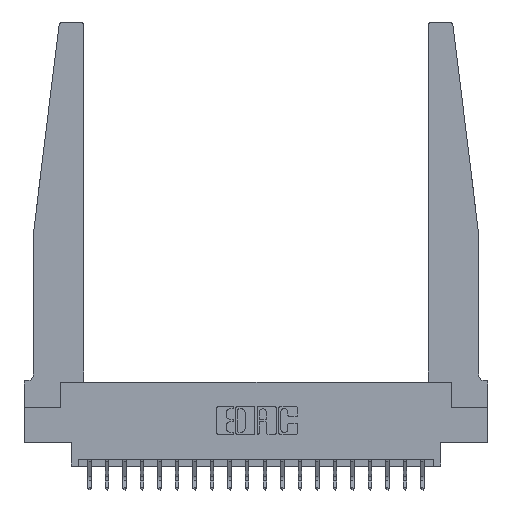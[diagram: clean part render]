
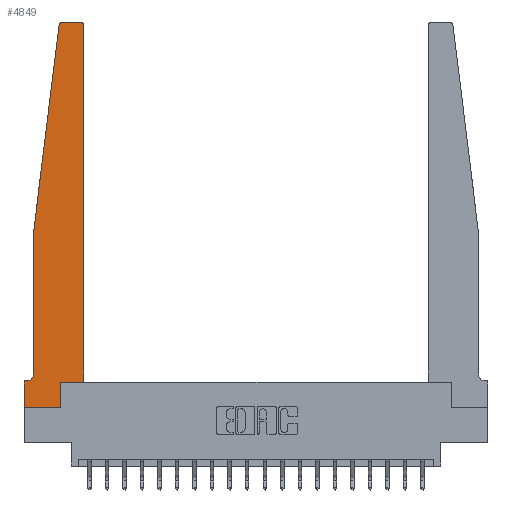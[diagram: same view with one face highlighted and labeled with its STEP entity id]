
A CAD part, top view. The second image highlights one B-rep face of the part: STEP entity #4849.
In plain terms, the highlighted planar face has unit normal (0, 0, 1).
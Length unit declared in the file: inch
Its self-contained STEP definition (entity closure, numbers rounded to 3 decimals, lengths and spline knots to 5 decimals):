
#12 = VERTEX_POINT ( 'NONE', #3323 ) ;
#208 = DIRECTION ( 'NONE',  ( -1., 0., 0. ) ) ;
#365 = VECTOR ( 'NONE', #12422, 39.37008 ) ;
#427 = LINE ( 'NONE', #16798, #15853 ) ;
#464 = VECTOR ( 'NONE', #8007, 39.37008 ) ;
#649 = ORIENTED_EDGE ( 'NONE', *, *, #1559, .T. ) ;
#778 = EDGE_CURVE ( 'NONE', #19258, #10017, #16864, .T. ) ;
#1355 = ORIENTED_EDGE ( 'NONE', *, *, #17358, .T. ) ;
#1365 = CARTESIAN_POINT ( 'NONE',  ( 0., 0., 0.37 ) ) ;
#1386 = VERTEX_POINT ( 'NONE', #12495 ) ;
#1539 = DIRECTION ( 'NONE',  ( -0.122, -0.992, 0. ) ) ;
#1559 = EDGE_CURVE ( 'NONE', #12, #13884, #9637, .T. ) ;
#1691 = EDGE_CURVE ( 'NONE', #13422, #20948, #4747, .T. ) ;
#1709 = CARTESIAN_POINT ( 'NONE',  ( 0., 0., 0.37 ) ) ;
#1996 = CARTESIAN_POINT ( 'NONE',  ( 0., 0.1875, 0.37 ) ) ;
#2006 = CARTESIAN_POINT ( 'NONE',  ( 0.27653, 2.72, 0.37 ) ) ;
#2047 = ORIENTED_EDGE ( 'NONE', *, *, #13869, .T. ) ;
#2962 = EDGE_CURVE ( 'NONE', #20948, #1386, #3175, .T. ) ;
#2971 = DIRECTION ( 'NONE',  ( -1., 0., 0. ) ) ;
#3175 = LINE ( 'NONE', #16484, #3456 ) ;
#3197 = CARTESIAN_POINT ( 'NONE',  ( 0.425, 0.18, 0.37 ) ) ;
#3222 = LINE ( 'NONE', #17869, #13721 ) ;
#3249 = EDGE_CURVE ( 'NONE', #1386, #19258, #3222, .T. ) ;
#3323 = CARTESIAN_POINT ( 'NONE',  ( 0., 0.1875, 0.37 ) ) ;
#3456 = VECTOR ( 'NONE', #1539, 39.37008 ) ;
#3509 = CARTESIAN_POINT ( 'NONE',  ( 0.27653, 2.75, 0.37 ) ) ;
#3515 = EDGE_CURVE ( 'NONE', #14419, #13780, #16507, .T. ) ;
#3523 = FACE_OUTER_BOUND ( 'NONE', #13510, .T. ) ;
#3864 = CIRCLE ( 'NONE', #15699, 0.03 ) ;
#4580 = ORIENTED_EDGE ( 'NONE', *, *, #1691, .T. ) ;
#4747 = CIRCLE ( 'NONE', #7854, 0.03 ) ;
#4849 = ADVANCED_FACE ( 'NONE', ( #3523 ), #8409, .T. ) ;
#5771 = ORIENTED_EDGE ( 'NONE', *, *, #17017, .T. ) ;
#5894 = EDGE_CURVE ( 'NONE', #12754, #19388, #3864, .T. ) ;
#5920 = CARTESIAN_POINT ( 'NONE',  ( 0.015, 0.2375, 0.37 ) ) ;
#6209 = CARTESIAN_POINT ( 'NONE',  ( 0.24675, 2.72367, 0.37 ) ) ;
#6405 = LINE ( 'NONE', #19714, #13813 ) ;
#6652 = ORIENTED_EDGE ( 'NONE', *, *, #778, .T. ) ;
#6830 = CARTESIAN_POINT ( 'NONE',  ( 0.425, 0.18, 0.37 ) ) ;
#6892 = CARTESIAN_POINT ( 'NONE',  ( 0.395, 2.75, 0.37 ) ) ;
#7793 = EDGE_CURVE ( 'NONE', #13884, #18957, #9132, .T. ) ;
#7854 = AXIS2_PLACEMENT_3D ( 'NONE', #2006, #14878, #21572 ) ;
#8007 = DIRECTION ( 'NONE',  ( 0., -1., 0. ) ) ;
#8185 = VECTOR ( 'NONE', #9976, 39.37008 ) ;
#8409 = PLANE ( 'NONE',  #14267 ) ;
#8577 = ORIENTED_EDGE ( 'NONE', *, *, #3515, .T. ) ;
#8632 = CARTESIAN_POINT ( 'NONE',  ( 0.2605, 0.18, 0.37 ) ) ;
#9132 = LINE ( 'NONE', #12530, #365 ) ;
#9637 = LINE ( 'NONE', #1365, #464 ) ;
#9976 = DIRECTION ( 'NONE',  ( 0., 1., 0. ) ) ;
#10017 = VERTEX_POINT ( 'NONE', #12161 ) ;
#10121 = CARTESIAN_POINT ( 'NONE',  ( 0.425, 0.18, 0.37 ) ) ;
#10492 = VECTOR ( 'NONE', #14661, 39.37008 ) ;
#11265 = CARTESIAN_POINT ( 'NONE',  ( 0.2605, 0., 0.37 ) ) ;
#11380 = CARTESIAN_POINT ( 'NONE',  ( 0.065, 0.1875, 0.37 ) ) ;
#11407 = DIRECTION ( 'NONE',  ( 0., 1., 0. ) ) ;
#11745 = VECTOR ( 'NONE', #16089, 39.37008 ) ;
#11844 = LINE ( 'NONE', #6830, #8185 ) ;
#11995 = ORIENTED_EDGE ( 'NONE', *, *, #5894, .T. ) ;
#12143 = ORIENTED_EDGE ( 'NONE', *, *, #14721, .T. ) ;
#12161 = CARTESIAN_POINT ( 'NONE',  ( 0.015, 0.1875, 0.37 ) ) ;
#12193 = DIRECTION ( 'NONE',  ( 0., 0., 1. ) ) ;
#12422 = DIRECTION ( 'NONE',  ( 1., 0., 0. ) ) ;
#12495 = CARTESIAN_POINT ( 'NONE',  ( 0.065, 1.25, 0.37 ) ) ;
#12530 = CARTESIAN_POINT ( 'NONE',  ( 0., 0., 0.37 ) ) ;
#12754 = VERTEX_POINT ( 'NONE', #17747 ) ;
#13422 = VERTEX_POINT ( 'NONE', #3509 ) ;
#13510 = EDGE_LOOP ( 'NONE', ( #12143, #4580, #20173, #17532, #6652, #1355, #649, #16756, #5771, #8577, #2047, #11995 ) ) ;
#13721 = VECTOR ( 'NONE', #16436, 39.37008 ) ;
#13780 = VERTEX_POINT ( 'NONE', #10121 ) ;
#13813 = VECTOR ( 'NONE', #11407, 39.37008 ) ;
#13869 = EDGE_CURVE ( 'NONE', #13780, #12754, #11844, .T. ) ;
#13884 = VERTEX_POINT ( 'NONE', #1709 ) ;
#14267 = AXIS2_PLACEMENT_3D ( 'NONE', #1996, #16725, #16837 ) ;
#14419 = VERTEX_POINT ( 'NONE', #8632 ) ;
#14661 = DIRECTION ( 'NONE',  ( 1., 0., 0. ) ) ;
#14721 = EDGE_CURVE ( 'NONE', #19388, #13422, #427, .T. ) ;
#14878 = DIRECTION ( 'NONE',  ( 0., 0., 1. ) ) ;
#15473 = DIRECTION ( 'NONE',  ( 1., 0., 0. ) ) ;
#15699 = AXIS2_PLACEMENT_3D ( 'NONE', #15802, #12193, #15473 ) ;
#15802 = CARTESIAN_POINT ( 'NONE',  ( 0.395, 2.72, 0.37 ) ) ;
#15853 = VECTOR ( 'NONE', #208, 39.37008 ) ;
#16089 = DIRECTION ( 'NONE',  ( -1., 0., 0. ) ) ;
#16183 = DIRECTION ( 'NONE',  ( 0., 0., -1. ) ) ;
#16436 = DIRECTION ( 'NONE',  ( 0., -1., 0. ) ) ;
#16484 = CARTESIAN_POINT ( 'NONE',  ( 0.065, 1.25, 0.37 ) ) ;
#16507 = LINE ( 'NONE', #3197, #10492 ) ;
#16725 = DIRECTION ( 'NONE',  ( 0., 0., 1. ) ) ;
#16756 = ORIENTED_EDGE ( 'NONE', *, *, #7793, .T. ) ;
#16798 = CARTESIAN_POINT ( 'NONE',  ( 0.25, 2.75, 0.37 ) ) ;
#16837 = DIRECTION ( 'NONE',  ( 1., 0., 0. ) ) ;
#16864 = CIRCLE ( 'NONE', #20384, 0.05 ) ;
#17017 = EDGE_CURVE ( 'NONE', #18957, #14419, #6405, .T. ) ;
#17358 = EDGE_CURVE ( 'NONE', #10017, #12, #21127, .T. ) ;
#17532 = ORIENTED_EDGE ( 'NONE', *, *, #3249, .T. ) ;
#17747 = CARTESIAN_POINT ( 'NONE',  ( 0.425, 2.72, 0.37 ) ) ;
#17869 = CARTESIAN_POINT ( 'NONE',  ( 0.065, 1.25, 0.37 ) ) ;
#18957 = VERTEX_POINT ( 'NONE', #11265 ) ;
#19258 = VERTEX_POINT ( 'NONE', #20215 ) ;
#19388 = VERTEX_POINT ( 'NONE', #6892 ) ;
#19714 = CARTESIAN_POINT ( 'NONE',  ( 0.2605, 0.18, 0.37 ) ) ;
#20173 = ORIENTED_EDGE ( 'NONE', *, *, #2962, .T. ) ;
#20215 = CARTESIAN_POINT ( 'NONE',  ( 0.065, 0.2375, 0.37 ) ) ;
#20384 = AXIS2_PLACEMENT_3D ( 'NONE', #5920, #16183, #2971 ) ;
#20948 = VERTEX_POINT ( 'NONE', #6209 ) ;
#21127 = LINE ( 'NONE', #11380, #11745 ) ;
#21572 = DIRECTION ( 'NONE',  ( 1., 0., 0. ) ) ;
